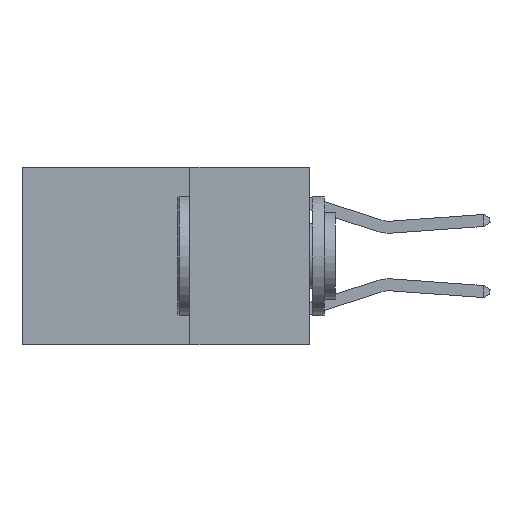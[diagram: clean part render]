
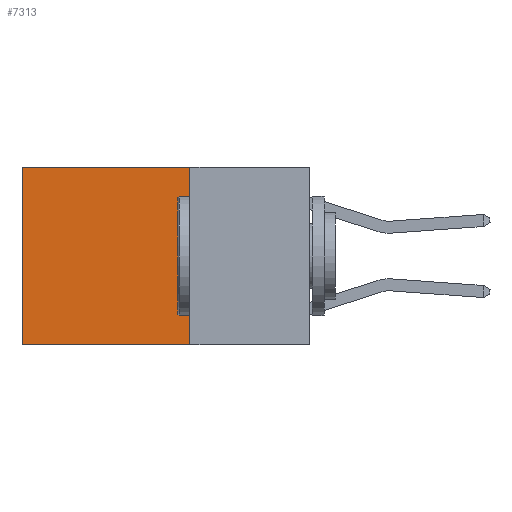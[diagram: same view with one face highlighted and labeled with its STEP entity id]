
A CAD part, left-side view. The second image highlights one B-rep face of the part: STEP entity #7313.
In plain terms, the highlighted planar face has unit normal (-1, 0, 0).
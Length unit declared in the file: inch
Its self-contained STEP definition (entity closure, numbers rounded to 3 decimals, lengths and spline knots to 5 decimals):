
#138 = VECTOR ( 'NONE', #13568, 39.37008 ) ;
#238 = CARTESIAN_POINT ( 'NONE',  ( 0.2625, 0.6, 0. ) ) ;
#574 = VERTEX_POINT ( 'NONE', #3177 ) ;
#997 = EDGE_LOOP ( 'NONE', ( #13243, #6067, #10711, #4418 ) ) ;
#1637 = AXIS2_PLACEMENT_3D ( 'NONE', #6964, #3383, #6729 ) ;
#1886 = PLANE ( 'NONE',  #1637 ) ;
#2092 = LINE ( 'NONE', #11577, #12077 ) ;
#2225 = CARTESIAN_POINT ( 'NONE',  ( 0.2625, 0.6, 0. ) ) ;
#3177 = CARTESIAN_POINT ( 'NONE',  ( 0.2625, 0.25, 0. ) ) ;
#3383 = DIRECTION ( 'NONE',  ( 1., 0., 0. ) ) ;
#3564 = DIRECTION ( 'NONE',  ( 0., 0., -1. ) ) ;
#4418 = ORIENTED_EDGE ( 'NONE', *, *, #10955, .T. ) ;
#5116 = LINE ( 'NONE', #8670, #9571 ) ;
#5366 = LINE ( 'NONE', #12464, #138 ) ;
#5951 = LINE ( 'NONE', #2225, #10036 ) ;
#6067 = ORIENTED_EDGE ( 'NONE', *, *, #7574, .F. ) ;
#6269 = VERTEX_POINT ( 'NONE', #6383 ) ;
#6383 = CARTESIAN_POINT ( 'NONE',  ( 0.2625, 0.6, -0.37 ) ) ;
#6535 = DIRECTION ( 'NONE',  ( 0., 0., -1. ) ) ;
#6621 = VERTEX_POINT ( 'NONE', #8831 ) ;
#6729 = DIRECTION ( 'NONE',  ( 0., 0., -1. ) ) ;
#6922 = DIRECTION ( 'NONE',  ( 0., 1., 0. ) ) ;
#6964 = CARTESIAN_POINT ( 'NONE',  ( 0.2625, 0.25, 0. ) ) ;
#7313 = ADVANCED_FACE ( 'NONE', ( #12951 ), #1886, .F. ) ;
#7574 = EDGE_CURVE ( 'NONE', #6621, #6269, #5366, .T. ) ;
#8670 = CARTESIAN_POINT ( 'NONE',  ( 0.2625, 0.25, 0. ) ) ;
#8831 = CARTESIAN_POINT ( 'NONE',  ( 0.2625, 0.25, -0.37 ) ) ;
#9571 = VECTOR ( 'NONE', #6535, 39.37008 ) ;
#10036 = VECTOR ( 'NONE', #3564, 39.37008 ) ;
#10238 = EDGE_CURVE ( 'NONE', #14073, #6269, #5951, .T. ) ;
#10711 = ORIENTED_EDGE ( 'NONE', *, *, #10817, .F. ) ;
#10817 = EDGE_CURVE ( 'NONE', #574, #6621, #5116, .T. ) ;
#10955 = EDGE_CURVE ( 'NONE', #574, #14073, #2092, .T. ) ;
#11577 = CARTESIAN_POINT ( 'NONE',  ( 0.2625, 0.25, 0. ) ) ;
#12077 = VECTOR ( 'NONE', #6922, 39.37008 ) ;
#12464 = CARTESIAN_POINT ( 'NONE',  ( 0.2625, 0.25, -0.37 ) ) ;
#12951 = FACE_OUTER_BOUND ( 'NONE', #997, .T. ) ;
#13243 = ORIENTED_EDGE ( 'NONE', *, *, #10238, .T. ) ;
#13568 = DIRECTION ( 'NONE',  ( 0., 1., 0. ) ) ;
#14073 = VERTEX_POINT ( 'NONE', #238 ) ;
